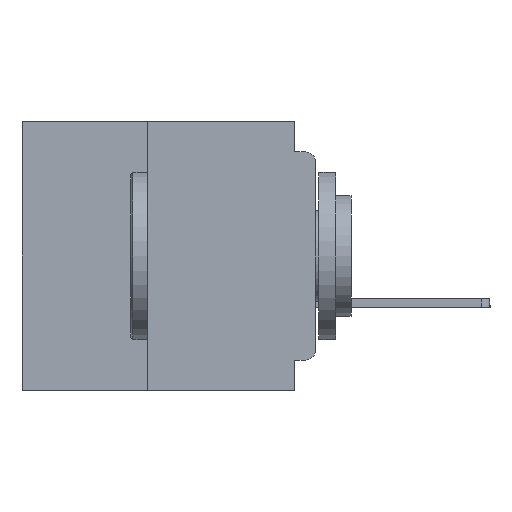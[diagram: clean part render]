
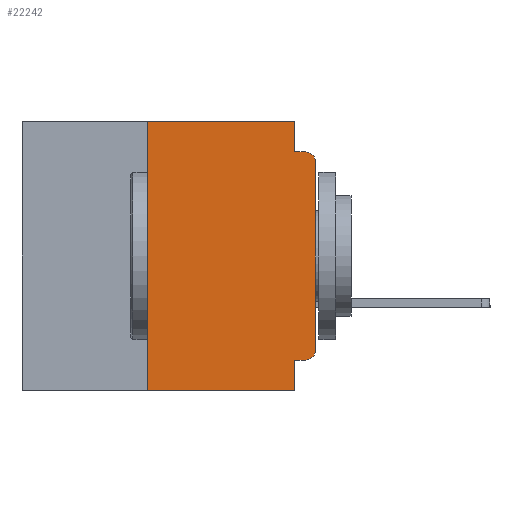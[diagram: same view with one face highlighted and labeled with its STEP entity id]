
A CAD part, left-side view. The second image highlights one B-rep face of the part: STEP entity #22242.
In plain terms, the highlighted planar face has unit normal (-1, 0, 0).
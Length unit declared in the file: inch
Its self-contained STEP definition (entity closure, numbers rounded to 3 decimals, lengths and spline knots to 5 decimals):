
#1591 = CARTESIAN_POINT ( 'NONE',  ( 0., 0.031, -0.355 ) ) ;
#1746 = CIRCLE ( 'NONE', #30342, 0.015 ) ;
#2084 = CARTESIAN_POINT ( 'NONE',  ( 0., 0., -0.045 ) ) ;
#2488 = DIRECTION ( 'NONE',  ( 0., 1., 0. ) ) ;
#3082 = CARTESIAN_POINT ( 'NONE',  ( 0., 0., -0.34 ) ) ;
#3277 = VECTOR ( 'NONE', #26000, 39.37008 ) ;
#3522 = CARTESIAN_POINT ( 'NONE',  ( 0., 0.437, -0.4 ) ) ;
#3633 = DIRECTION ( 'NONE',  ( 0., 0., -1. ) ) ;
#3839 = CARTESIAN_POINT ( 'NONE',  ( 0., 0., 0. ) ) ;
#4265 = DIRECTION ( 'NONE',  ( 0., 0., -1. ) ) ;
#4620 = VECTOR ( 'NONE', #7061, 39.37008 ) ;
#5331 = AXIS2_PLACEMENT_3D ( 'NONE', #18941, #26269, #4265 ) ;
#5615 = ORIENTED_EDGE ( 'NONE', *, *, #33090, .T. ) ;
#6089 = EDGE_CURVE ( 'NONE', #38796, #7184, #28125, .T. ) ;
#7061 = DIRECTION ( 'NONE',  ( 0., -1., 0. ) ) ;
#7184 = VERTEX_POINT ( 'NONE', #24430 ) ;
#8444 = VERTEX_POINT ( 'NONE', #1591 ) ;
#9915 = CARTESIAN_POINT ( 'NONE',  ( 0., 0., -0.355 ) ) ;
#10525 = VECTOR ( 'NONE', #47023, 39.37008 ) ;
#11978 = LINE ( 'NONE', #19651, #42204 ) ;
#12437 = CARTESIAN_POINT ( 'NONE',  ( 0., 0.031, -0.4 ) ) ;
#12474 = CARTESIAN_POINT ( 'NONE',  ( 0., 0.015, -0.34 ) ) ;
#13509 = EDGE_CURVE ( 'NONE', #7184, #42483, #33607, .T. ) ;
#13971 = EDGE_LOOP ( 'NONE', ( #5615, #19272, #19031, #31197, #15566, #27642, #33527, #21217, #22905, #41508 ) ) ;
#14919 = EDGE_CURVE ( 'NONE', #28640, #18898, #31143, .T. ) ;
#15000 = CARTESIAN_POINT ( 'NONE',  ( 0., 0.015, -0.045 ) ) ;
#15566 = ORIENTED_EDGE ( 'NONE', *, *, #27749, .F. ) ;
#15617 = EDGE_CURVE ( 'NONE', #26478, #42483, #1746, .T. ) ;
#16175 = DIRECTION ( 'NONE',  ( 0., 0., -1. ) ) ;
#16231 = CARTESIAN_POINT ( 'NONE',  ( 0., 0.25, -0.4 ) ) ;
#17586 = CARTESIAN_POINT ( 'NONE',  ( 0., 0.437, 0. ) ) ;
#18427 = VECTOR ( 'NONE', #28140, 39.37008 ) ;
#18898 = VERTEX_POINT ( 'NONE', #29903 ) ;
#18941 = CARTESIAN_POINT ( 'NONE',  ( 0., 0.437, 0. ) ) ;
#19031 = ORIENTED_EDGE ( 'NONE', *, *, #13509, .F. ) ;
#19272 = ORIENTED_EDGE ( 'NONE', *, *, #15617, .T. ) ;
#19651 = CARTESIAN_POINT ( 'NONE',  ( 0., 0.031, -0.4 ) ) ;
#21217 = ORIENTED_EDGE ( 'NONE', *, *, #38892, .F. ) ;
#22242 = ADVANCED_FACE ( 'NONE', ( #30463 ), #40776, .F. ) ;
#22663 = CARTESIAN_POINT ( 'NONE',  ( 0., 0.031, 0. ) ) ;
#22905 = ORIENTED_EDGE ( 'NONE', *, *, #32267, .F. ) ;
#23510 = CIRCLE ( 'NONE', #30460, 0.015 ) ;
#24430 = CARTESIAN_POINT ( 'NONE',  ( 0., 0.031, -0.045 ) ) ;
#25626 = DIRECTION ( 'NONE',  ( -1., 0., 0. ) ) ;
#26000 = DIRECTION ( 'NONE',  ( 0., 0., 1. ) ) ;
#26269 = DIRECTION ( 'NONE',  ( 1., 0., 0. ) ) ;
#26478 = VERTEX_POINT ( 'NONE', #42348 ) ;
#27642 = ORIENTED_EDGE ( 'NONE', *, *, #14919, .F. ) ;
#27749 = EDGE_CURVE ( 'NONE', #18898, #38796, #33995, .T. ) ;
#28125 = LINE ( 'NONE', #28603, #18427 ) ;
#28140 = DIRECTION ( 'NONE',  ( 0., 0., -1. ) ) ;
#28603 = CARTESIAN_POINT ( 'NONE',  ( 0., 0.031, 0. ) ) ;
#28640 = VERTEX_POINT ( 'NONE', #16231 ) ;
#29903 = CARTESIAN_POINT ( 'NONE',  ( 0., 0.25, 0. ) ) ;
#30342 = AXIS2_PLACEMENT_3D ( 'NONE', #45781, #25626, #3633 ) ;
#30356 = VECTOR ( 'NONE', #2488, 39.37008 ) ;
#30460 = AXIS2_PLACEMENT_3D ( 'NONE', #12474, #37991, #16175 ) ;
#30463 = FACE_OUTER_BOUND ( 'NONE', #13971, .T. ) ;
#31143 = LINE ( 'NONE', #43366, #10525 ) ;
#31197 = ORIENTED_EDGE ( 'NONE', *, *, #6089, .F. ) ;
#31518 = LINE ( 'NONE', #9915, #30356 ) ;
#32267 = EDGE_CURVE ( 'NONE', #43763, #8444, #31518, .T. ) ;
#32438 = VECTOR ( 'NONE', #42239, 39.37008 ) ;
#33090 = EDGE_CURVE ( 'NONE', #36113, #26478, #42210, .T. ) ;
#33527 = ORIENTED_EDGE ( 'NONE', *, *, #36703, .T. ) ;
#33607 = LINE ( 'NONE', #2084, #32438 ) ;
#33995 = LINE ( 'NONE', #17586, #45867 ) ;
#36113 = VERTEX_POINT ( 'NONE', #3082 ) ;
#36703 = EDGE_CURVE ( 'NONE', #28640, #40427, #40140, .T. ) ;
#37222 = EDGE_CURVE ( 'NONE', #43763, #36113, #23510, .T. ) ;
#37991 = DIRECTION ( 'NONE',  ( -1., 0., 0. ) ) ;
#38005 = CARTESIAN_POINT ( 'NONE',  ( 0., 0.015, -0.355 ) ) ;
#38796 = VERTEX_POINT ( 'NONE', #22663 ) ;
#38892 = EDGE_CURVE ( 'NONE', #8444, #40427, #11978, .T. ) ;
#40140 = LINE ( 'NONE', #3522, #4620 ) ;
#40427 = VERTEX_POINT ( 'NONE', #12437 ) ;
#40776 = PLANE ( 'NONE',  #5331 ) ;
#41508 = ORIENTED_EDGE ( 'NONE', *, *, #37222, .T. ) ;
#42204 = VECTOR ( 'NONE', #45135, 39.37008 ) ;
#42210 = LINE ( 'NONE', #3839, #3277 ) ;
#42239 = DIRECTION ( 'NONE',  ( 0., -1., 0. ) ) ;
#42348 = CARTESIAN_POINT ( 'NONE',  ( 0., 0., -0.06 ) ) ;
#42483 = VERTEX_POINT ( 'NONE', #15000 ) ;
#43034 = DIRECTION ( 'NONE',  ( 0., -1., 0. ) ) ;
#43366 = CARTESIAN_POINT ( 'NONE',  ( 0., 0.25, -0.4 ) ) ;
#43763 = VERTEX_POINT ( 'NONE', #38005 ) ;
#45135 = DIRECTION ( 'NONE',  ( 0., 0., -1. ) ) ;
#45781 = CARTESIAN_POINT ( 'NONE',  ( 0., 0.015, -0.06 ) ) ;
#45867 = VECTOR ( 'NONE', #43034, 39.37008 ) ;
#47023 = DIRECTION ( 'NONE',  ( 0., 0., 1. ) ) ;
